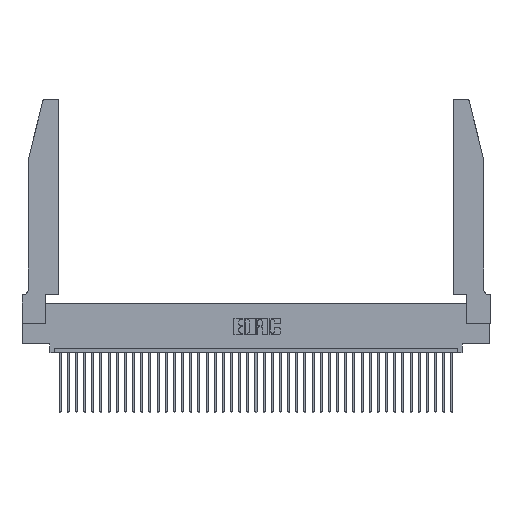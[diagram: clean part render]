
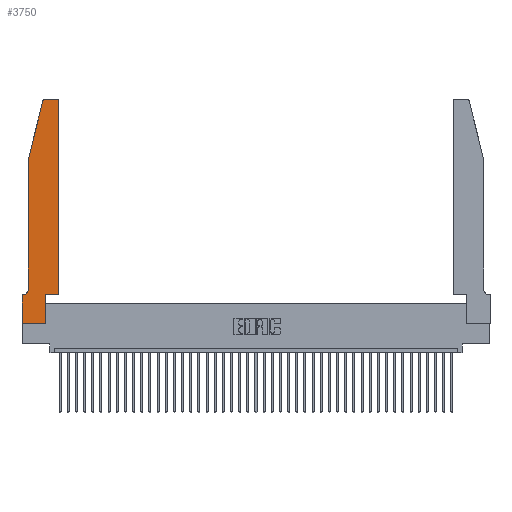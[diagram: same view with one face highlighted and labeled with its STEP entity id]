
A CAD part, top view. The second image highlights one B-rep face of the part: STEP entity #3750.
In plain terms, the highlighted planar face has unit normal (0, 0, 1).
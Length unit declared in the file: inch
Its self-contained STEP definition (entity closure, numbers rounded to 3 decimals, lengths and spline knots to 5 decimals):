
#758 = EDGE_CURVE ( 'NONE', #13654, #7324, #7638, .T. ) ;
#1032 = VECTOR ( 'NONE', #13533, 39.37008 ) ;
#2176 = AXIS2_PLACEMENT_3D ( 'NONE', #23392, #4441, #26541 ) ;
#2246 = CARTESIAN_POINT ( 'NONE',  ( 0., 0., 0.37 ) ) ;
#2347 = EDGE_CURVE ( 'NONE', #12900, #26743, #17975, .T. ) ;
#3098 = VECTOR ( 'NONE', #35592, 39.37008 ) ;
#3482 = EDGE_CURVE ( 'NONE', #35096, #19950, #13855, .T. ) ;
#3750 = ADVANCED_FACE ( 'NONE', ( #20833 ), #28508, .T. ) ;
#4441 = DIRECTION ( 'NONE',  ( 0., 0., 1. ) ) ;
#4596 = CARTESIAN_POINT ( 'NONE',  ( 0.2865, 0.35, 0.37 ) ) ;
#4885 = CARTESIAN_POINT ( 'NONE',  ( 0.4205, 2.75, 0.37 ) ) ;
#4953 = CARTESIAN_POINT ( 'NONE',  ( 0., 0., 0.37 ) ) ;
#5486 = VECTOR ( 'NONE', #30966, 39.37008 ) ;
#5626 = CARTESIAN_POINT ( 'NONE',  ( 0.4505, 0.35, 0.37 ) ) ;
#5920 = CARTESIAN_POINT ( 'NONE',  ( 0.0055, 0.35, 0.37 ) ) ;
#6846 = EDGE_CURVE ( 'NONE', #8693, #22493, #14115, .T. ) ;
#6942 = LINE ( 'NONE', #2246, #5486 ) ;
#7324 = VERTEX_POINT ( 'NONE', #5920 ) ;
#7430 = LINE ( 'NONE', #38740, #1032 ) ;
#7638 = CIRCLE ( 'NONE', #7822, 0.07 ) ;
#7822 = AXIS2_PLACEMENT_3D ( 'NONE', #8189, #30263, #11339 ) ;
#8189 = CARTESIAN_POINT ( 'NONE',  ( 0.0055, 0.42, 0.37 ) ) ;
#8503 = EDGE_LOOP ( 'NONE', ( #8755, #10111, #30353, #24795, #12297, #20000, #25853, #40102, #19926, #12568, #24200, #26072 ) ) ;
#8693 = VERTEX_POINT ( 'NONE', #16377 ) ;
#8755 = ORIENTED_EDGE ( 'NONE', *, *, #18794, .T. ) ;
#8925 = LINE ( 'NONE', #18919, #21771 ) ;
#9401 = LINE ( 'NONE', #24173, #40026 ) ;
#9975 = DIRECTION ( 'NONE',  ( 1., 0., 0. ) ) ;
#10111 = ORIENTED_EDGE ( 'NONE', *, *, #3482, .T. ) ;
#10131 = DIRECTION ( 'NONE',  ( 0., 1., 0. ) ) ;
#10528 = VERTEX_POINT ( 'NONE', #4953 ) ;
#11339 = DIRECTION ( 'NONE',  ( -1., 0., 0. ) ) ;
#11370 = LINE ( 'NONE', #30344, #15389 ) ;
#11811 = DIRECTION ( 'NONE',  ( 1., 0., 0. ) ) ;
#12297 = ORIENTED_EDGE ( 'NONE', *, *, #758, .T. ) ;
#12568 = ORIENTED_EDGE ( 'NONE', *, *, #31332, .T. ) ;
#12900 = VERTEX_POINT ( 'NONE', #33985 ) ;
#13302 = CARTESIAN_POINT ( 'NONE',  ( 0.4505, 2.72, 0.37 ) ) ;
#13423 = AXIS2_PLACEMENT_3D ( 'NONE', #36751, #30747, #11811 ) ;
#13533 = DIRECTION ( 'NONE',  ( 0., -1., 0. ) ) ;
#13654 = VERTEX_POINT ( 'NONE', #38285 ) ;
#13855 = CIRCLE ( 'NONE', #13423, 0.03 ) ;
#13976 = LINE ( 'NONE', #5626, #20415 ) ;
#14115 = LINE ( 'NONE', #16651, #21541 ) ;
#14561 = DIRECTION ( 'NONE',  ( -0.239, -0.971, 0. ) ) ;
#15049 = CARTESIAN_POINT ( 'NONE',  ( 0.25487, 2.72718, 0.37 ) ) ;
#15389 = VECTOR ( 'NONE', #17951, 39.37008 ) ;
#16377 = CARTESIAN_POINT ( 'NONE',  ( 0.4505, 0.35, 0.37 ) ) ;
#16651 = CARTESIAN_POINT ( 'NONE',  ( 0.4505, 0.35, 0.37 ) ) ;
#17951 = DIRECTION ( 'NONE',  ( 1., 0., 0. ) ) ;
#17975 = LINE ( 'NONE', #35863, #3098 ) ;
#18158 = EDGE_CURVE ( 'NONE', #7324, #23983, #9401, .T. ) ;
#18368 = DIRECTION ( 'NONE',  ( 1., 0., 0. ) ) ;
#18794 = EDGE_CURVE ( 'NONE', #23611, #35096, #8925, .T. ) ;
#18919 = CARTESIAN_POINT ( 'NONE',  ( 0.2605, 2.75, 0.37 ) ) ;
#19680 = CARTESIAN_POINT ( 'NONE',  ( 0.284, 2.75, 0.37 ) ) ;
#19926 = ORIENTED_EDGE ( 'NONE', *, *, #2347, .T. ) ;
#19950 = VERTEX_POINT ( 'NONE', #15049 ) ;
#20000 = ORIENTED_EDGE ( 'NONE', *, *, #18158, .T. ) ;
#20415 = VECTOR ( 'NONE', #18368, 39.37008 ) ;
#20833 = FACE_OUTER_BOUND ( 'NONE', #8503, .T. ) ;
#21541 = VECTOR ( 'NONE', #10131, 39.37008 ) ;
#21771 = VECTOR ( 'NONE', #28391, 39.37008 ) ;
#22048 = CARTESIAN_POINT ( 'NONE',  ( 0., 0.35, 0.37 ) ) ;
#22493 = VERTEX_POINT ( 'NONE', #13302 ) ;
#23392 = CARTESIAN_POINT ( 'NONE',  ( 0.4205, 2.72, 0.37 ) ) ;
#23499 = EDGE_CURVE ( 'NONE', #38530, #13654, #7430, .T. ) ;
#23611 = VERTEX_POINT ( 'NONE', #4885 ) ;
#23983 = VERTEX_POINT ( 'NONE', #27148 ) ;
#24155 = CIRCLE ( 'NONE', #2176, 0.03 ) ;
#24173 = CARTESIAN_POINT ( 'NONE',  ( 0.0755, 0.35, 0.37 ) ) ;
#24200 = ORIENTED_EDGE ( 'NONE', *, *, #6846, .T. ) ;
#24795 = ORIENTED_EDGE ( 'NONE', *, *, #23499, .T. ) ;
#25542 = EDGE_CURVE ( 'NONE', #23983, #10528, #6942, .T. ) ;
#25704 = EDGE_CURVE ( 'NONE', #10528, #12900, #11370, .T. ) ;
#25853 = ORIENTED_EDGE ( 'NONE', *, *, #25542, .T. ) ;
#26072 = ORIENTED_EDGE ( 'NONE', *, *, #26735, .T. ) ;
#26541 = DIRECTION ( 'NONE',  ( 1., 0., 0. ) ) ;
#26735 = EDGE_CURVE ( 'NONE', #22493, #23611, #24155, .T. ) ;
#26743 = VERTEX_POINT ( 'NONE', #4596 ) ;
#26792 = CARTESIAN_POINT ( 'NONE',  ( 0.0755, 2., 0.37 ) ) ;
#27148 = CARTESIAN_POINT ( 'NONE',  ( 0., 0.35, 0.37 ) ) ;
#27309 = LINE ( 'NONE', #26792, #29764 ) ;
#27329 = DIRECTION ( 'NONE',  ( -1., 0., 0. ) ) ;
#27726 = AXIS2_PLACEMENT_3D ( 'NONE', #22048, #38130, #9975 ) ;
#28391 = DIRECTION ( 'NONE',  ( -1., 0., 0. ) ) ;
#28508 = PLANE ( 'NONE',  #27726 ) ;
#29764 = VECTOR ( 'NONE', #14561, 39.37008 ) ;
#30263 = DIRECTION ( 'NONE',  ( 0., 0., -1. ) ) ;
#30344 = CARTESIAN_POINT ( 'NONE',  ( 0., 0., 0.37 ) ) ;
#30353 = ORIENTED_EDGE ( 'NONE', *, *, #36569, .T. ) ;
#30747 = DIRECTION ( 'NONE',  ( 0., 0., 1. ) ) ;
#30966 = DIRECTION ( 'NONE',  ( 0., -1., 0. ) ) ;
#31332 = EDGE_CURVE ( 'NONE', #26743, #8693, #13976, .T. ) ;
#33985 = CARTESIAN_POINT ( 'NONE',  ( 0.2865, 0., 0.37 ) ) ;
#35096 = VERTEX_POINT ( 'NONE', #19680 ) ;
#35556 = CARTESIAN_POINT ( 'NONE',  ( 0.0755, 2., 0.37 ) ) ;
#35592 = DIRECTION ( 'NONE',  ( 0., 1., 0. ) ) ;
#35863 = CARTESIAN_POINT ( 'NONE',  ( 0.2865, 0.35, 0.37 ) ) ;
#36569 = EDGE_CURVE ( 'NONE', #19950, #38530, #27309, .T. ) ;
#36751 = CARTESIAN_POINT ( 'NONE',  ( 0.284, 2.72, 0.37 ) ) ;
#38130 = DIRECTION ( 'NONE',  ( 0., 0., 1. ) ) ;
#38285 = CARTESIAN_POINT ( 'NONE',  ( 0.0755, 0.42, 0.37 ) ) ;
#38530 = VERTEX_POINT ( 'NONE', #35556 ) ;
#38740 = CARTESIAN_POINT ( 'NONE',  ( 0.0755, 2., 0.37 ) ) ;
#40026 = VECTOR ( 'NONE', #27329, 39.37008 ) ;
#40102 = ORIENTED_EDGE ( 'NONE', *, *, #25704, .T. ) ;
